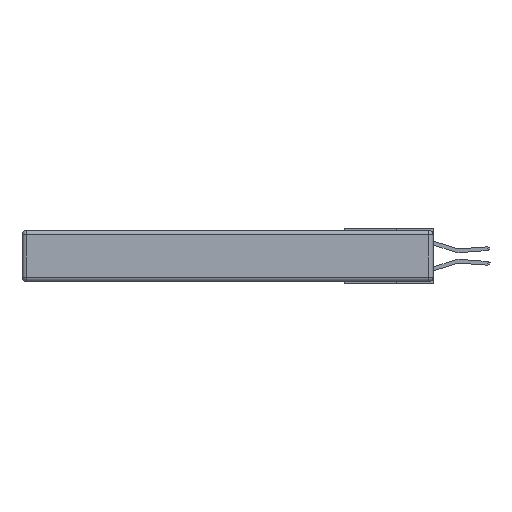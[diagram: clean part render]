
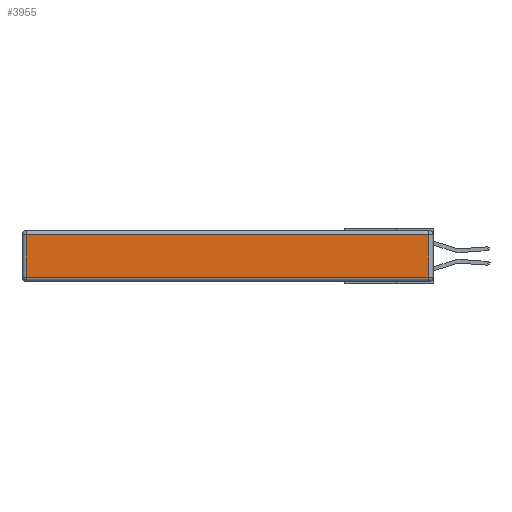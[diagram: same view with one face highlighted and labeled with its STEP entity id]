
A CAD part, left-side view. The second image highlights one B-rep face of the part: STEP entity #3955.
In plain terms, the highlighted planar face has unit normal (-1, 0, 0).
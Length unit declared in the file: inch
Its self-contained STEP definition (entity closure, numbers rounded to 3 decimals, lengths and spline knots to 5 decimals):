
#553 = DIRECTION ( 'NONE',  ( -1., 0., 0. ) ) ;
#2701 = ORIENTED_EDGE ( 'NONE', *, *, #18934, .T. ) ;
#3204 = DIRECTION ( 'NONE',  ( 0., 1., 0. ) ) ;
#3730 = LINE ( 'NONE', #23823, #5024 ) ;
#3955 = ADVANCED_FACE ( 'NONE', ( #21623 ), #23536, .T. ) ;
#4816 = DIRECTION ( 'NONE',  ( 0., 0., 1. ) ) ;
#4914 = CARTESIAN_POINT ( 'NONE',  ( 0., 2.72, -0.343 ) ) ;
#5024 = VECTOR ( 'NONE', #3204, 39.37008 ) ;
#6629 = CARTESIAN_POINT ( 'NONE',  ( 0., 0.03, -0.313 ) ) ;
#7203 = CARTESIAN_POINT ( 'NONE',  ( 0., 2.72, -0.313 ) ) ;
#8309 = VERTEX_POINT ( 'NONE', #18672 ) ;
#10449 = EDGE_CURVE ( 'NONE', #26090, #19253, #23988, .T. ) ;
#10698 = ORIENTED_EDGE ( 'NONE', *, *, #25478, .T. ) ;
#10861 = EDGE_CURVE ( 'NONE', #19253, #8309, #3730, .T. ) ;
#11172 = EDGE_LOOP ( 'NONE', ( #2701, #16519, #20531, #10698 ) ) ;
#13071 = CARTESIAN_POINT ( 'NONE',  ( 0., 0., -0.343 ) ) ;
#14017 = AXIS2_PLACEMENT_3D ( 'NONE', #13071, #553, #4816 ) ;
#14527 = VECTOR ( 'NONE', #18261, 39.37008 ) ;
#15067 = DIRECTION ( 'NONE',  ( 0., -1., 0. ) ) ;
#16001 = CARTESIAN_POINT ( 'NONE',  ( 0., 0.03, -0.343 ) ) ;
#16519 = ORIENTED_EDGE ( 'NONE', *, *, #10449, .T. ) ;
#17688 = LINE ( 'NONE', #24021, #21967 ) ;
#18261 = DIRECTION ( 'NONE',  ( 0., 0., 1. ) ) ;
#18672 = CARTESIAN_POINT ( 'NONE',  ( 0., 2.72, -0.03 ) ) ;
#18934 = EDGE_CURVE ( 'NONE', #24576, #26090, #17688, .T. ) ;
#19253 = VERTEX_POINT ( 'NONE', #19494 ) ;
#19494 = CARTESIAN_POINT ( 'NONE',  ( 0., 0.03, -0.03 ) ) ;
#20531 = ORIENTED_EDGE ( 'NONE', *, *, #10861, .T. ) ;
#20678 = VECTOR ( 'NONE', #21927, 39.37008 ) ;
#21623 = FACE_OUTER_BOUND ( 'NONE', #11172, .T. ) ;
#21693 = LINE ( 'NONE', #4914, #20678 ) ;
#21927 = DIRECTION ( 'NONE',  ( 0., 0., -1. ) ) ;
#21967 = VECTOR ( 'NONE', #15067, 39.37008 ) ;
#23536 = PLANE ( 'NONE',  #14017 ) ;
#23823 = CARTESIAN_POINT ( 'NONE',  ( 0., 2.75, -0.03 ) ) ;
#23988 = LINE ( 'NONE', #16001, #14527 ) ;
#24021 = CARTESIAN_POINT ( 'NONE',  ( 0., 0., -0.313 ) ) ;
#24576 = VERTEX_POINT ( 'NONE', #7203 ) ;
#25478 = EDGE_CURVE ( 'NONE', #8309, #24576, #21693, .T. ) ;
#26090 = VERTEX_POINT ( 'NONE', #6629 ) ;
